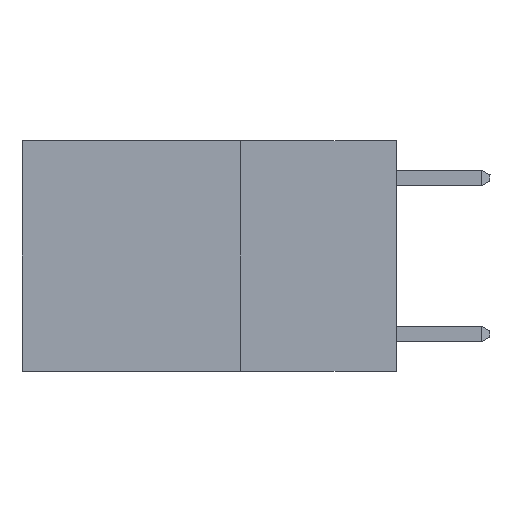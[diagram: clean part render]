
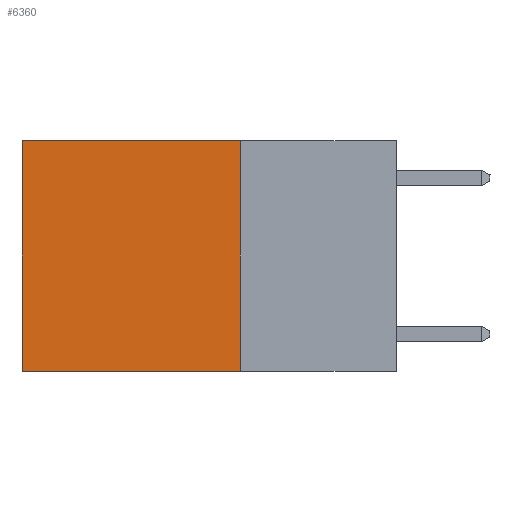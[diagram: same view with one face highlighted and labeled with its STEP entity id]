
A CAD part, left-side view. The second image highlights one B-rep face of the part: STEP entity #6360.
In plain terms, the highlighted planar face has unit normal (-1, 0, 0).
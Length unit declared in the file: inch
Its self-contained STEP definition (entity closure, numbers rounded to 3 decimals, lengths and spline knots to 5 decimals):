
#249 = VERTEX_POINT ( 'NONE', #3228 ) ;
#376 = ORIENTED_EDGE ( 'NONE', *, *, #2502, .F. ) ;
#392 = EDGE_CURVE ( 'NONE', #249, #3915, #3511, .T. ) ;
#1310 = ORIENTED_EDGE ( 'NONE', *, *, #2342, .F. ) ;
#1695 = DIRECTION ( 'NONE',  ( 0., 1., 0. ) ) ;
#1971 = DIRECTION ( 'NONE',  ( 0., 0., -1. ) ) ;
#2342 = EDGE_CURVE ( 'NONE', #5888, #3915, #2664, .T. ) ;
#2502 = EDGE_CURVE ( 'NONE', #2736, #5888, #4566, .T. ) ;
#2664 = LINE ( 'NONE', #7928, #8750 ) ;
#2736 = VERTEX_POINT ( 'NONE', #9490 ) ;
#3095 = CARTESIAN_POINT ( 'NONE',  ( 0.2625, 0.25, -0.37 ) ) ;
#3228 = CARTESIAN_POINT ( 'NONE',  ( 0.2625, 0.6, 0. ) ) ;
#3314 = DIRECTION ( 'NONE',  ( 0., 1., 0. ) ) ;
#3470 = VECTOR ( 'NONE', #5822, 39.37008 ) ;
#3483 = EDGE_CURVE ( 'NONE', #2736, #249, #9185, .T. ) ;
#3511 = LINE ( 'NONE', #6512, #3470 ) ;
#3833 = CARTESIAN_POINT ( 'NONE',  ( 0.2625, 0.25, 0. ) ) ;
#3915 = VERTEX_POINT ( 'NONE', #5428 ) ;
#4566 = LINE ( 'NONE', #3833, #5302 ) ;
#5302 = VECTOR ( 'NONE', #1971, 39.37008 ) ;
#5309 = DIRECTION ( 'NONE',  ( 0., 0., -1. ) ) ;
#5428 = CARTESIAN_POINT ( 'NONE',  ( 0.2625, 0.6, -0.37 ) ) ;
#5437 = CARTESIAN_POINT ( 'NONE',  ( 0.2625, 0.25, 0. ) ) ;
#5822 = DIRECTION ( 'NONE',  ( 0., 0., -1. ) ) ;
#5888 = VERTEX_POINT ( 'NONE', #3095 ) ;
#5907 = ORIENTED_EDGE ( 'NONE', *, *, #392, .T. ) ;
#6044 = PLANE ( 'NONE',  #8224 ) ;
#6360 = ADVANCED_FACE ( 'NONE', ( #7671 ), #6044, .F. ) ;
#6512 = CARTESIAN_POINT ( 'NONE',  ( 0.2625, 0.6, 0. ) ) ;
#7290 = ORIENTED_EDGE ( 'NONE', *, *, #3483, .T. ) ;
#7671 = FACE_OUTER_BOUND ( 'NONE', #9640, .T. ) ;
#7928 = CARTESIAN_POINT ( 'NONE',  ( 0.2625, 0.25, -0.37 ) ) ;
#8224 = AXIS2_PLACEMENT_3D ( 'NONE', #9049, #9105, #5309 ) ;
#8624 = VECTOR ( 'NONE', #1695, 39.37008 ) ;
#8750 = VECTOR ( 'NONE', #3314, 39.37008 ) ;
#9049 = CARTESIAN_POINT ( 'NONE',  ( 0.2625, 0.25, 0. ) ) ;
#9105 = DIRECTION ( 'NONE',  ( 1., 0., 0. ) ) ;
#9185 = LINE ( 'NONE', #5437, #8624 ) ;
#9490 = CARTESIAN_POINT ( 'NONE',  ( 0.2625, 0.25, 0. ) ) ;
#9640 = EDGE_LOOP ( 'NONE', ( #5907, #1310, #376, #7290 ) ) ;
